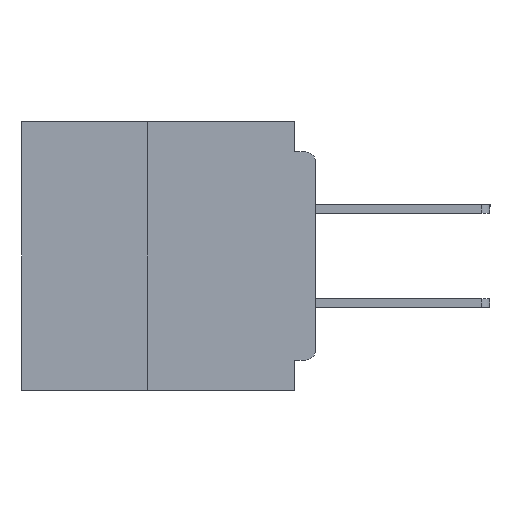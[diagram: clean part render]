
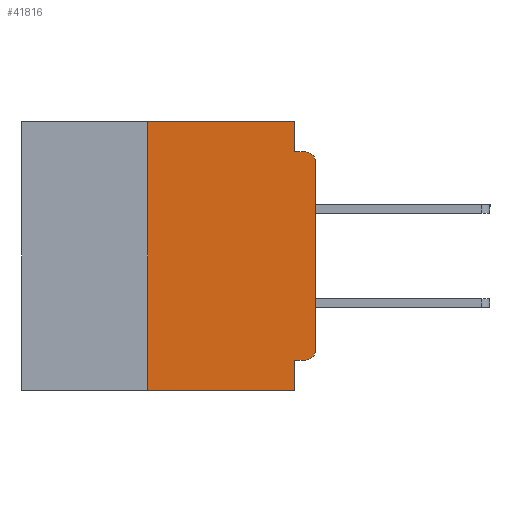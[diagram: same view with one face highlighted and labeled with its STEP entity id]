
A CAD part, left-side view. The second image highlights one B-rep face of the part: STEP entity #41816.
In plain terms, the highlighted planar face has unit normal (-1, 0, 0).
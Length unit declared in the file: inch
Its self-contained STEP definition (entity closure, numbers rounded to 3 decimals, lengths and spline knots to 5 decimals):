
#538 = VECTOR ( 'NONE', #23515, 39.37008 ) ;
#1144 = VERTEX_POINT ( 'NONE', #27411 ) ;
#1765 = CIRCLE ( 'NONE', #31305, 0.015 ) ;
#2716 = ORIENTED_EDGE ( 'NONE', *, *, #22656, .F. ) ;
#3152 = VECTOR ( 'NONE', #29298, 39.37008 ) ;
#3307 = EDGE_CURVE ( 'NONE', #5049, #1144, #19567, .T. ) ;
#4963 = DIRECTION ( 'NONE',  ( 0., 0., -1. ) ) ;
#5049 = VERTEX_POINT ( 'NONE', #43881 ) ;
#5168 = CARTESIAN_POINT ( 'NONE',  ( 0., 0.015, -0.34 ) ) ;
#6124 = CARTESIAN_POINT ( 'NONE',  ( 0., 0.25, -0.4 ) ) ;
#6446 = CARTESIAN_POINT ( 'NONE',  ( 0., 0.25, -0.4 ) ) ;
#6539 = CARTESIAN_POINT ( 'NONE',  ( 0., 0.25, 0. ) ) ;
#7844 = CARTESIAN_POINT ( 'NONE',  ( 0., 0.031, -0.4 ) ) ;
#8039 = EDGE_CURVE ( 'NONE', #35372, #45811, #36304, .T. ) ;
#8225 = CARTESIAN_POINT ( 'NONE',  ( 0., 0.015, -0.06 ) ) ;
#8322 = CARTESIAN_POINT ( 'NONE',  ( 0., 0., -0.355 ) ) ;
#8735 = DIRECTION ( 'NONE',  ( 0., 0., -1. ) ) ;
#8916 = LINE ( 'NONE', #8322, #36129 ) ;
#9108 = DIRECTION ( 'NONE',  ( 0., -1., 0. ) ) ;
#9160 = VERTEX_POINT ( 'NONE', #32128 ) ;
#11622 = DIRECTION ( 'NONE',  ( 0., 0., -1. ) ) ;
#11839 = DIRECTION ( 'NONE',  ( 0., 0., -1. ) ) ;
#12209 = EDGE_CURVE ( 'NONE', #18836, #5049, #32587, .T. ) ;
#12420 = VECTOR ( 'NONE', #39829, 39.37008 ) ;
#12858 = ORIENTED_EDGE ( 'NONE', *, *, #8039, .F. ) ;
#12875 = ORIENTED_EDGE ( 'NONE', *, *, #36846, .T. ) ;
#13286 = ORIENTED_EDGE ( 'NONE', *, *, #23745, .T. ) ;
#16071 = EDGE_LOOP ( 'NONE', ( #44089, #13286, #19300, #20670, #17578, #19561, #12875, #12858, #2716, #17266 ) ) ;
#17146 = DIRECTION ( 'NONE',  ( 0., 0., 1. ) ) ;
#17266 = ORIENTED_EDGE ( 'NONE', *, *, #45838, .T. ) ;
#17578 = ORIENTED_EDGE ( 'NONE', *, *, #18234, .F. ) ;
#18234 = EDGE_CURVE ( 'NONE', #45008, #18836, #21462, .T. ) ;
#18746 = CARTESIAN_POINT ( 'NONE',  ( 0., 0., 0. ) ) ;
#18836 = VERTEX_POINT ( 'NONE', #30807 ) ;
#19300 = ORIENTED_EDGE ( 'NONE', *, *, #3307, .F. ) ;
#19401 = LINE ( 'NONE', #30458, #538 ) ;
#19561 = ORIENTED_EDGE ( 'NONE', *, *, #29074, .F. ) ;
#19567 = LINE ( 'NONE', #38367, #27921 ) ;
#20670 = ORIENTED_EDGE ( 'NONE', *, *, #12209, .F. ) ;
#21462 = LINE ( 'NONE', #26890, #40288 ) ;
#22656 = EDGE_CURVE ( 'NONE', #37391, #35372, #8916, .T. ) ;
#22724 = PLANE ( 'NONE',  #28574 ) ;
#23515 = DIRECTION ( 'NONE',  ( 0., -1., 0. ) ) ;
#23628 = CARTESIAN_POINT ( 'NONE',  ( 0., 0.015, -0.355 ) ) ;
#23745 = EDGE_CURVE ( 'NONE', #9160, #1144, #45449, .T. ) ;
#25918 = CARTESIAN_POINT ( 'NONE',  ( 0., 0.031, 0. ) ) ;
#26323 = DIRECTION ( 'NONE',  ( 1., 0., 0. ) ) ;
#26890 = CARTESIAN_POINT ( 'NONE',  ( 0., 0.437, 0. ) ) ;
#27383 = EDGE_CURVE ( 'NONE', #41065, #9160, #31295, .T. ) ;
#27411 = CARTESIAN_POINT ( 'NONE',  ( 0., 0.015, -0.045 ) ) ;
#27921 = VECTOR ( 'NONE', #35490, 39.37008 ) ;
#28574 = AXIS2_PLACEMENT_3D ( 'NONE', #33234, #26323, #4963 ) ;
#29074 = EDGE_CURVE ( 'NONE', #31505, #45008, #45555, .T. ) ;
#29298 = DIRECTION ( 'NONE',  ( 0., 0., -1. ) ) ;
#30042 = DIRECTION ( 'NONE',  ( -1., 0., 0. ) ) ;
#30458 = CARTESIAN_POINT ( 'NONE',  ( 0., 0.437, -0.4 ) ) ;
#30807 = CARTESIAN_POINT ( 'NONE',  ( 0., 0.031, 0. ) ) ;
#31295 = LINE ( 'NONE', #18746, #12420 ) ;
#31305 = AXIS2_PLACEMENT_3D ( 'NONE', #5168, #30042, #8735 ) ;
#31505 = VERTEX_POINT ( 'NONE', #6124 ) ;
#32128 = CARTESIAN_POINT ( 'NONE',  ( 0., 0., -0.06 ) ) ;
#32587 = LINE ( 'NONE', #25918, #3152 ) ;
#32676 = FACE_OUTER_BOUND ( 'NONE', #16071, .T. ) ;
#33082 = DIRECTION ( 'NONE',  ( -1., 0., 0. ) ) ;
#33234 = CARTESIAN_POINT ( 'NONE',  ( 0., 0.437, 0. ) ) ;
#35372 = VERTEX_POINT ( 'NONE', #36855 ) ;
#35490 = DIRECTION ( 'NONE',  ( 0., -1., 0. ) ) ;
#36129 = VECTOR ( 'NONE', #36752, 39.37008 ) ;
#36304 = LINE ( 'NONE', #7844, #44531 ) ;
#36752 = DIRECTION ( 'NONE',  ( 0., 1., 0. ) ) ;
#36846 = EDGE_CURVE ( 'NONE', #31505, #45811, #19401, .T. ) ;
#36855 = CARTESIAN_POINT ( 'NONE',  ( 0., 0.031, -0.355 ) ) ;
#37391 = VERTEX_POINT ( 'NONE', #23628 ) ;
#38367 = CARTESIAN_POINT ( 'NONE',  ( 0., 0., -0.045 ) ) ;
#39829 = DIRECTION ( 'NONE',  ( 0., 0., 1. ) ) ;
#40288 = VECTOR ( 'NONE', #9108, 39.37008 ) ;
#41065 = VERTEX_POINT ( 'NONE', #45743 ) ;
#41499 = AXIS2_PLACEMENT_3D ( 'NONE', #8225, #33082, #11839 ) ;
#41816 = ADVANCED_FACE ( 'NONE', ( #32676 ), #22724, .F. ) ;
#43756 = CARTESIAN_POINT ( 'NONE',  ( 0., 0.031, -0.4 ) ) ;
#43881 = CARTESIAN_POINT ( 'NONE',  ( 0., 0.031, -0.045 ) ) ;
#44089 = ORIENTED_EDGE ( 'NONE', *, *, #27383, .T. ) ;
#44447 = VECTOR ( 'NONE', #17146, 39.37008 ) ;
#44531 = VECTOR ( 'NONE', #11622, 39.37008 ) ;
#45008 = VERTEX_POINT ( 'NONE', #6539 ) ;
#45449 = CIRCLE ( 'NONE', #41499, 0.015 ) ;
#45555 = LINE ( 'NONE', #6446, #44447 ) ;
#45743 = CARTESIAN_POINT ( 'NONE',  ( 0., 0., -0.34 ) ) ;
#45811 = VERTEX_POINT ( 'NONE', #43756 ) ;
#45838 = EDGE_CURVE ( 'NONE', #37391, #41065, #1765, .T. ) ;
